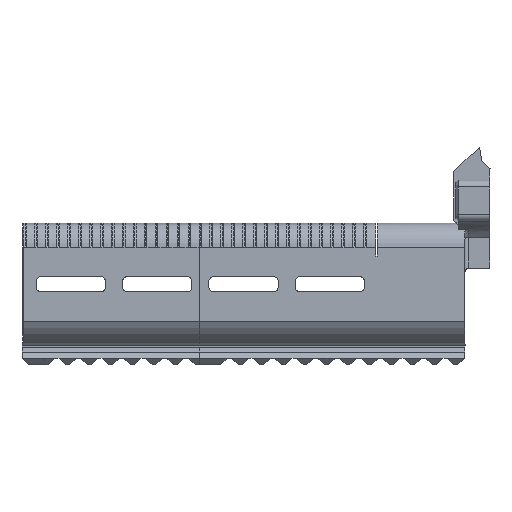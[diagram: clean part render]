
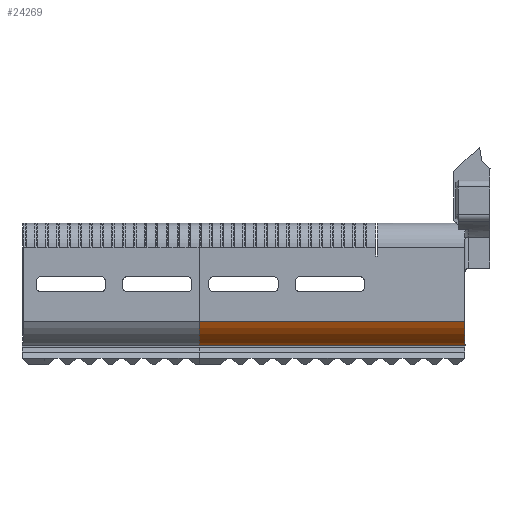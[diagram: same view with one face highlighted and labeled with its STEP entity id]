
A CAD part, front view. The second image highlights one B-rep face of the part: STEP entity #24269.
In plain terms, the highlighted cylindrical face has radius 21.012 mm (diameter 42.024 mm), a partial arc.
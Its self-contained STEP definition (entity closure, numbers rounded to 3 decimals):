
#2124=FACE_OUTER_BOUND('',#3595,.T.);
#3595=EDGE_LOOP('',(#20673,#20674,#20675,#20676));
#4744=CIRCLE('',#26369,21.012);
#4778=CIRCLE('',#26410,21.012);
#6916=LINE('',#44180,#9276);
#6962=LINE('',#44288,#9322);
#9276=VECTOR('',#32092,1000.);
#9322=VECTOR('',#32156,1000.);
#11485=VERTEX_POINT('',#43921);
#11486=VERTEX_POINT('',#43923);
#11608=VERTEX_POINT('',#44179);
#11661=VERTEX_POINT('',#44287);
#14584=EDGE_CURVE('',#11486,#11485,#4744,.T.);
#14712=EDGE_CURVE('',#11486,#11608,#6916,.T.);
#14766=EDGE_CURVE('',#11485,#11661,#6962,.T.);
#14767=EDGE_CURVE('',#11608,#11661,#4778,.T.);
#20673=ORIENTED_EDGE('',*,*,#14584,.T.);
#20674=ORIENTED_EDGE('',*,*,#14766,.T.);
#20675=ORIENTED_EDGE('',*,*,#14767,.F.);
#20676=ORIENTED_EDGE('',*,*,#14712,.F.);
#23199=CYLINDRICAL_SURFACE('',#26409,21.012);
#24269=ADVANCED_FACE('',(#2124),#23199,.T.);
#26369=AXIS2_PLACEMENT_3D('',#43924,#31926,#31927);
#26409=AXIS2_PLACEMENT_3D('',#44286,#32154,#32155);
#26410=AXIS2_PLACEMENT_3D('',#44289,#32157,#32158);
#31926=DIRECTION('center_axis',(1.,0.,0.));
#31927=DIRECTION('ref_axis',(0.,1.,0.));
#32092=DIRECTION('',(1.,0.,0.));
#32154=DIRECTION('center_axis',(1.,0.,0.));
#32155=DIRECTION('ref_axis',(0.,1.,0.));
#32156=DIRECTION('',(1.,0.,0.));
#32157=DIRECTION('center_axis',(1.,0.,0.));
#32158=DIRECTION('ref_axis',(0.,-1.,0.));
#43921=CARTESIAN_POINT('',(-39.195,157.051,91.096));
#43923=CARTESIAN_POINT('',(-39.195,169.751,79.933));
#43924=CARTESIAN_POINT('Origin',(-39.195,150.701,71.067));
#44179=CARTESIAN_POINT('',(83.995,169.751,79.933));
#44180=CARTESIAN_POINT('',(43.355,169.751,79.933));
#44286=CARTESIAN_POINT('Origin',(43.355,150.701,71.067));
#44287=CARTESIAN_POINT('',(83.995,157.051,91.096));
#44288=CARTESIAN_POINT('',(43.355,157.051,91.096));
#44289=CARTESIAN_POINT('Origin',(83.995,150.701,71.067));
